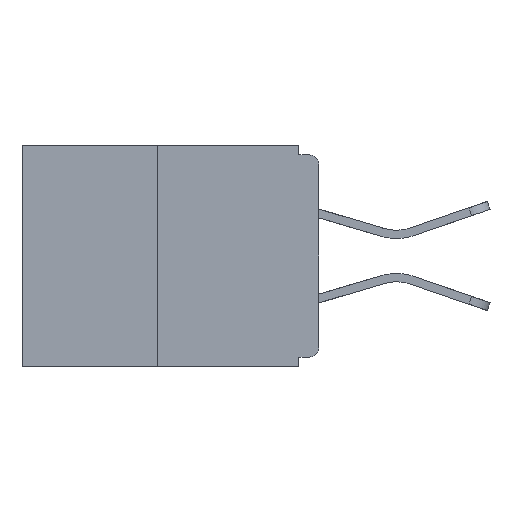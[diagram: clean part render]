
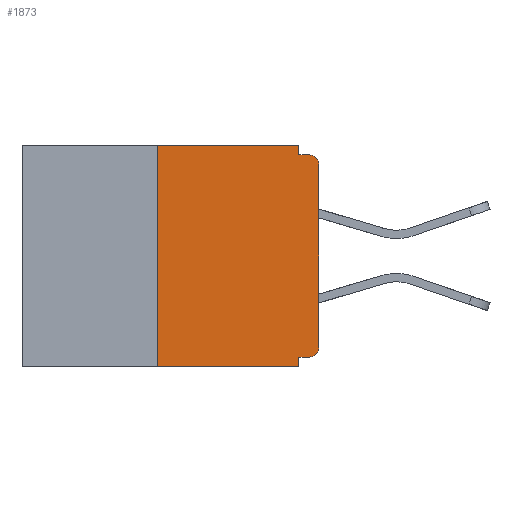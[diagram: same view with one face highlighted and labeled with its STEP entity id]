
A CAD part, left-side view. The second image highlights one B-rep face of the part: STEP entity #1873.
In plain terms, the highlighted planar face has unit normal (-1, 0, 0).
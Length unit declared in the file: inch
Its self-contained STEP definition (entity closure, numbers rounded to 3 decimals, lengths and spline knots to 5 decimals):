
#371 = VERTEX_POINT ( 'NONE', #14150 ) ;
#568 = CARTESIAN_POINT ( 'NONE',  ( 0., 0.015, -0.328 ) ) ;
#593 = CARTESIAN_POINT ( 'NONE',  ( 0., 0.46, 0. ) ) ;
#951 = VECTOR ( 'NONE', #1832, 39.37008 ) ;
#1172 = LINE ( 'NONE', #21710, #22961 ) ;
#1359 = VECTOR ( 'NONE', #17435, 39.37008 ) ;
#1440 = ORIENTED_EDGE ( 'NONE', *, *, #8693, .F. ) ;
#1517 = VECTOR ( 'NONE', #3253, 39.37008 ) ;
#1659 = DIRECTION ( 'NONE',  ( -1., 0., 0. ) ) ;
#1832 = DIRECTION ( 'NONE',  ( 0., 0., -1. ) ) ;
#1846 = AXIS2_PLACEMENT_3D ( 'NONE', #593, #18662, #9695 ) ;
#1873 = ADVANCED_FACE ( 'NONE', ( #7924 ), #18581, .F. ) ;
#2355 = VERTEX_POINT ( 'NONE', #19227 ) ;
#2383 = LINE ( 'NONE', #8719, #1517 ) ;
#2437 = ORIENTED_EDGE ( 'NONE', *, *, #12896, .F. ) ;
#2634 = VECTOR ( 'NONE', #4506, 39.37008 ) ;
#3253 = DIRECTION ( 'NONE',  ( 0., 0., 1. ) ) ;
#3401 = CARTESIAN_POINT ( 'NONE',  ( 0., 0.015, -0.015 ) ) ;
#3853 = CARTESIAN_POINT ( 'NONE',  ( 0., 0.25, 0. ) ) ;
#3907 = VECTOR ( 'NONE', #22802, 39.37008 ) ;
#4268 = ORIENTED_EDGE ( 'NONE', *, *, #19815, .T. ) ;
#4348 = VERTEX_POINT ( 'NONE', #12283 ) ;
#4428 = LINE ( 'NONE', #5928, #16510 ) ;
#4506 = DIRECTION ( 'NONE',  ( 0., 1., 0. ) ) ;
#4717 = VERTEX_POINT ( 'NONE', #13271 ) ;
#4723 = CARTESIAN_POINT ( 'NONE',  ( 0., 0.46, 0. ) ) ;
#5385 = CARTESIAN_POINT ( 'NONE',  ( 0., 0.031, -0.343 ) ) ;
#5499 = EDGE_CURVE ( 'NONE', #371, #19517, #6386, .T. ) ;
#5542 = VERTEX_POINT ( 'NONE', #15809 ) ;
#5928 = CARTESIAN_POINT ( 'NONE',  ( 0., 0., 0. ) ) ;
#6099 = EDGE_LOOP ( 'NONE', ( #2437, #7100, #15115, #6908, #9867, #9667, #4268, #23278, #1440, #15920 ) ) ;
#6217 = CARTESIAN_POINT ( 'NONE',  ( 0., 0.031, -0.343 ) ) ;
#6386 = CIRCLE ( 'NONE', #22178, 0.015 ) ;
#6396 = VERTEX_POINT ( 'NONE', #3853 ) ;
#6908 = ORIENTED_EDGE ( 'NONE', *, *, #7507, .F. ) ;
#7100 = ORIENTED_EDGE ( 'NONE', *, *, #19479, .F. ) ;
#7507 = EDGE_CURVE ( 'NONE', #4348, #8266, #13608, .T. ) ;
#7823 = EDGE_CURVE ( 'NONE', #19252, #4348, #16421, .T. ) ;
#7924 = FACE_OUTER_BOUND ( 'NONE', #6099, .T. ) ;
#8075 = CARTESIAN_POINT ( 'NONE',  ( 0., 0., -0.328 ) ) ;
#8266 = VERTEX_POINT ( 'NONE', #6217 ) ;
#8358 = DIRECTION ( 'NONE',  ( 0., -1., 0. ) ) ;
#8420 = CARTESIAN_POINT ( 'NONE',  ( 0., 0.031, 0. ) ) ;
#8639 = CARTESIAN_POINT ( 'NONE',  ( 0., 0.015, -0.03 ) ) ;
#8693 = EDGE_CURVE ( 'NONE', #4717, #19517, #1172, .T. ) ;
#8719 = CARTESIAN_POINT ( 'NONE',  ( 0., 0.25, 0. ) ) ;
#9667 = ORIENTED_EDGE ( 'NONE', *, *, #15242, .T. ) ;
#9695 = DIRECTION ( 'NONE',  ( 0., 0., -1. ) ) ;
#9867 = ORIENTED_EDGE ( 'NONE', *, *, #7823, .F. ) ;
#10282 = CARTESIAN_POINT ( 'NONE',  ( 0., 0.46, -0.343 ) ) ;
#10654 = EDGE_CURVE ( 'NONE', #2355, #8266, #18291, .T. ) ;
#10877 = DIRECTION ( 'NONE',  ( 0., -1., 0. ) ) ;
#11337 = EDGE_CURVE ( 'NONE', #5542, #4717, #15987, .T. ) ;
#12283 = CARTESIAN_POINT ( 'NONE',  ( 0., 0.031, -0.328 ) ) ;
#12896 = EDGE_CURVE ( 'NONE', #6396, #5542, #18206, .T. ) ;
#13271 = CARTESIAN_POINT ( 'NONE',  ( 0., 0.031, -0.015 ) ) ;
#13384 = VECTOR ( 'NONE', #8358, 39.37008 ) ;
#13608 = LINE ( 'NONE', #5385, #951 ) ;
#14150 = CARTESIAN_POINT ( 'NONE',  ( 0., 0., -0.03 ) ) ;
#14492 = CARTESIAN_POINT ( 'NONE',  ( 0., 0., -0.313 ) ) ;
#15115 = ORIENTED_EDGE ( 'NONE', *, *, #10654, .T. ) ;
#15242 = EDGE_CURVE ( 'NONE', #19252, #19127, #18530, .T. ) ;
#15809 = CARTESIAN_POINT ( 'NONE',  ( 0., 0.031, 0. ) ) ;
#15845 = DIRECTION ( 'NONE',  ( 0., 0., -1. ) ) ;
#15920 = ORIENTED_EDGE ( 'NONE', *, *, #11337, .F. ) ;
#15929 = CARTESIAN_POINT ( 'NONE',  ( 0., 0.015, -0.313 ) ) ;
#15987 = LINE ( 'NONE', #8420, #3907 ) ;
#16001 = DIRECTION ( 'NONE',  ( -1., 0., 0. ) ) ;
#16421 = LINE ( 'NONE', #8075, #2634 ) ;
#16510 = VECTOR ( 'NONE', #18611, 39.37008 ) ;
#17435 = DIRECTION ( 'NONE',  ( 0., -1., 0. ) ) ;
#18206 = LINE ( 'NONE', #4723, #13384 ) ;
#18291 = LINE ( 'NONE', #10282, #1359 ) ;
#18530 = CIRCLE ( 'NONE', #23066, 0.015 ) ;
#18581 = PLANE ( 'NONE',  #1846 ) ;
#18611 = DIRECTION ( 'NONE',  ( 0., 0., 1. ) ) ;
#18662 = DIRECTION ( 'NONE',  ( 1., 0., 0. ) ) ;
#19127 = VERTEX_POINT ( 'NONE', #14492 ) ;
#19227 = CARTESIAN_POINT ( 'NONE',  ( 0., 0.25, -0.343 ) ) ;
#19252 = VERTEX_POINT ( 'NONE', #568 ) ;
#19479 = EDGE_CURVE ( 'NONE', #2355, #6396, #2383, .T. ) ;
#19517 = VERTEX_POINT ( 'NONE', #3401 ) ;
#19815 = EDGE_CURVE ( 'NONE', #19127, #371, #4428, .T. ) ;
#21710 = CARTESIAN_POINT ( 'NONE',  ( 0., 0., -0.015 ) ) ;
#22178 = AXIS2_PLACEMENT_3D ( 'NONE', #8639, #1659, #23250 ) ;
#22802 = DIRECTION ( 'NONE',  ( 0., 0., -1. ) ) ;
#22961 = VECTOR ( 'NONE', #10877, 39.37008 ) ;
#23066 = AXIS2_PLACEMENT_3D ( 'NONE', #15929, #16001, #15845 ) ;
#23250 = DIRECTION ( 'NONE',  ( 0., 0., -1. ) ) ;
#23278 = ORIENTED_EDGE ( 'NONE', *, *, #5499, .T. ) ;
